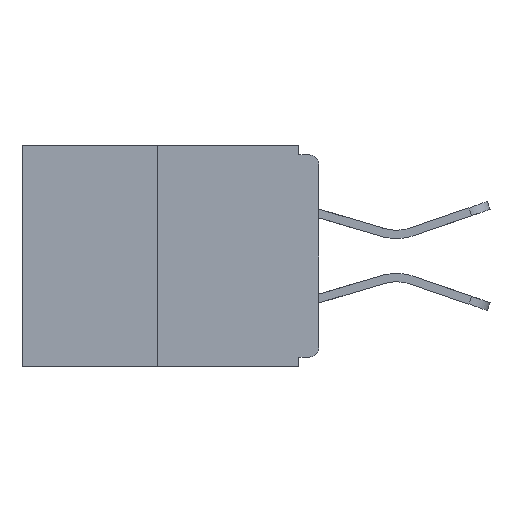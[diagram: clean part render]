
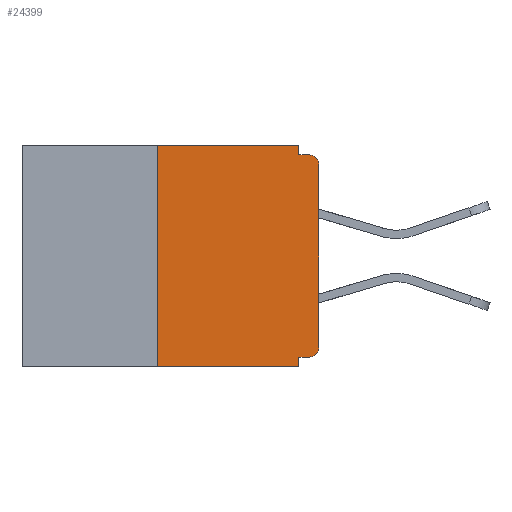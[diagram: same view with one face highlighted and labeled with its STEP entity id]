
A CAD part, left-side view. The second image highlights one B-rep face of the part: STEP entity #24399.
In plain terms, the highlighted planar face has unit normal (-1, 0, 0).
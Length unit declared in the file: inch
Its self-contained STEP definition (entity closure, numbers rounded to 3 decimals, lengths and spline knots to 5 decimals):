
#1397 = VERTEX_POINT ( 'NONE', #19082 ) ;
#1749 = VERTEX_POINT ( 'NONE', #22923 ) ;
#1788 = DIRECTION ( 'NONE',  ( 0., 0., -1. ) ) ;
#2247 = VECTOR ( 'NONE', #5165, 39.37008 ) ;
#2702 = EDGE_CURVE ( 'NONE', #28048, #22150, #17705, .T. ) ;
#2738 = DIRECTION ( 'NONE',  ( 0., 0., 1. ) ) ;
#2947 = EDGE_CURVE ( 'NONE', #25550, #29652, #5237, .T. ) ;
#3746 = EDGE_CURVE ( 'NONE', #1749, #10654, #16520, .T. ) ;
#4570 = ORIENTED_EDGE ( 'NONE', *, *, #2702, .F. ) ;
#4919 = LINE ( 'NONE', #8852, #24931 ) ;
#5165 = DIRECTION ( 'NONE',  ( 0., 1., 0. ) ) ;
#5237 = CIRCLE ( 'NONE', #24449, 0.015 ) ;
#6305 = VECTOR ( 'NONE', #8846, 39.37008 ) ;
#6596 = DIRECTION ( 'NONE',  ( -1., 0., 0. ) ) ;
#6628 = CARTESIAN_POINT ( 'NONE',  ( 0., 0.46, 0. ) ) ;
#6824 = DIRECTION ( 'NONE',  ( 1., 0., 0. ) ) ;
#7145 = LINE ( 'NONE', #29511, #24987 ) ;
#7838 = EDGE_LOOP ( 'NONE', ( #16862, #23389, #20081, #11694, #21338, #14393, #10015, #11213, #13718, #4570 ) ) ;
#8846 = DIRECTION ( 'NONE',  ( 0., -1., 0. ) ) ;
#8852 = CARTESIAN_POINT ( 'NONE',  ( 0., 0.25, 0. ) ) ;
#10015 = ORIENTED_EDGE ( 'NONE', *, *, #14027, .T. ) ;
#10208 = EDGE_CURVE ( 'NONE', #1749, #14489, #4919, .T. ) ;
#10329 = DIRECTION ( 'NONE',  ( 0., 0., -1. ) ) ;
#10654 = VERTEX_POINT ( 'NONE', #12079 ) ;
#11213 = ORIENTED_EDGE ( 'NONE', *, *, #2947, .T. ) ;
#11694 = ORIENTED_EDGE ( 'NONE', *, *, #17436, .F. ) ;
#11818 = CARTESIAN_POINT ( 'NONE',  ( 0., 0.015, -0.328 ) ) ;
#12079 = CARTESIAN_POINT ( 'NONE',  ( 0., 0.031, -0.343 ) ) ;
#12590 = CARTESIAN_POINT ( 'NONE',  ( 0., 0., -0.313 ) ) ;
#13718 = ORIENTED_EDGE ( 'NONE', *, *, #18125, .F. ) ;
#14027 = EDGE_CURVE ( 'NONE', #26965, #25550, #21138, .T. ) ;
#14182 = CARTESIAN_POINT ( 'NONE',  ( 0., 0.031, 0. ) ) ;
#14393 = ORIENTED_EDGE ( 'NONE', *, *, #23036, .T. ) ;
#14489 = VERTEX_POINT ( 'NONE', #25852 ) ;
#14754 = LINE ( 'NONE', #20647, #26398 ) ;
#14923 = VECTOR ( 'NONE', #2738, 39.37008 ) ;
#15770 = CARTESIAN_POINT ( 'NONE',  ( 0., 0.031, -0.343 ) ) ;
#16520 = LINE ( 'NONE', #22791, #6305 ) ;
#16862 = ORIENTED_EDGE ( 'NONE', *, *, #22563, .F. ) ;
#17436 = EDGE_CURVE ( 'NONE', #1397, #10654, #18502, .T. ) ;
#17705 = LINE ( 'NONE', #20652, #29680 ) ;
#18125 = EDGE_CURVE ( 'NONE', #22150, #29652, #7145, .T. ) ;
#18143 = DIRECTION ( 'NONE',  ( 0., 0., -1. ) ) ;
#18202 = DIRECTION ( 'NONE',  ( 0., -1., 0. ) ) ;
#18502 = LINE ( 'NONE', #15770, #21760 ) ;
#19045 = FACE_OUTER_BOUND ( 'NONE', #7838, .T. ) ;
#19082 = CARTESIAN_POINT ( 'NONE',  ( 0., 0.031, -0.328 ) ) ;
#19151 = AXIS2_PLACEMENT_3D ( 'NONE', #22689, #6596, #22592 ) ;
#19724 = DIRECTION ( 'NONE',  ( -1., 0., 0. ) ) ;
#20081 = ORIENTED_EDGE ( 'NONE', *, *, #3746, .T. ) ;
#20647 = CARTESIAN_POINT ( 'NONE',  ( 0., 0.46, 0. ) ) ;
#20652 = CARTESIAN_POINT ( 'NONE',  ( 0., 0.031, 0. ) ) ;
#21138 = LINE ( 'NONE', #21304, #14923 ) ;
#21304 = CARTESIAN_POINT ( 'NONE',  ( 0., 0., 0. ) ) ;
#21338 = ORIENTED_EDGE ( 'NONE', *, *, #24653, .F. ) ;
#21690 = CARTESIAN_POINT ( 'NONE',  ( 0., 0., -0.328 ) ) ;
#21760 = VECTOR ( 'NONE', #1788, 39.37008 ) ;
#22150 = VERTEX_POINT ( 'NONE', #28538 ) ;
#22472 = VERTEX_POINT ( 'NONE', #11818 ) ;
#22563 = EDGE_CURVE ( 'NONE', #14489, #28048, #14754, .T. ) ;
#22592 = DIRECTION ( 'NONE',  ( 0., 0., -1. ) ) ;
#22689 = CARTESIAN_POINT ( 'NONE',  ( 0., 0.015, -0.313 ) ) ;
#22737 = CARTESIAN_POINT ( 'NONE',  ( 0., 0.015, -0.015 ) ) ;
#22791 = CARTESIAN_POINT ( 'NONE',  ( 0., 0.46, -0.343 ) ) ;
#22884 = DIRECTION ( 'NONE',  ( 0., 0., -1. ) ) ;
#22923 = CARTESIAN_POINT ( 'NONE',  ( 0., 0.25, -0.343 ) ) ;
#23016 = PLANE ( 'NONE',  #28306 ) ;
#23036 = EDGE_CURVE ( 'NONE', #22472, #26965, #25719, .T. ) ;
#23389 = ORIENTED_EDGE ( 'NONE', *, *, #10208, .F. ) ;
#24399 = ADVANCED_FACE ( 'NONE', ( #19045 ), #23016, .F. ) ;
#24449 = AXIS2_PLACEMENT_3D ( 'NONE', #26729, #19724, #10329 ) ;
#24534 = DIRECTION ( 'NONE',  ( 0., -1., 0. ) ) ;
#24653 = EDGE_CURVE ( 'NONE', #22472, #1397, #27019, .T. ) ;
#24931 = VECTOR ( 'NONE', #29414, 39.37008 ) ;
#24987 = VECTOR ( 'NONE', #24534, 39.37008 ) ;
#24990 = CARTESIAN_POINT ( 'NONE',  ( 0., 0., -0.03 ) ) ;
#25550 = VERTEX_POINT ( 'NONE', #24990 ) ;
#25719 = CIRCLE ( 'NONE', #19151, 0.015 ) ;
#25852 = CARTESIAN_POINT ( 'NONE',  ( 0., 0.25, 0. ) ) ;
#26398 = VECTOR ( 'NONE', #18202, 39.37008 ) ;
#26729 = CARTESIAN_POINT ( 'NONE',  ( 0., 0.015, -0.03 ) ) ;
#26965 = VERTEX_POINT ( 'NONE', #12590 ) ;
#27019 = LINE ( 'NONE', #21690, #2247 ) ;
#28048 = VERTEX_POINT ( 'NONE', #14182 ) ;
#28306 = AXIS2_PLACEMENT_3D ( 'NONE', #6628, #6824, #18143 ) ;
#28538 = CARTESIAN_POINT ( 'NONE',  ( 0., 0.031, -0.015 ) ) ;
#29414 = DIRECTION ( 'NONE',  ( 0., 0., 1. ) ) ;
#29511 = CARTESIAN_POINT ( 'NONE',  ( 0., 0., -0.015 ) ) ;
#29652 = VERTEX_POINT ( 'NONE', #22737 ) ;
#29680 = VECTOR ( 'NONE', #22884, 39.37008 ) ;
